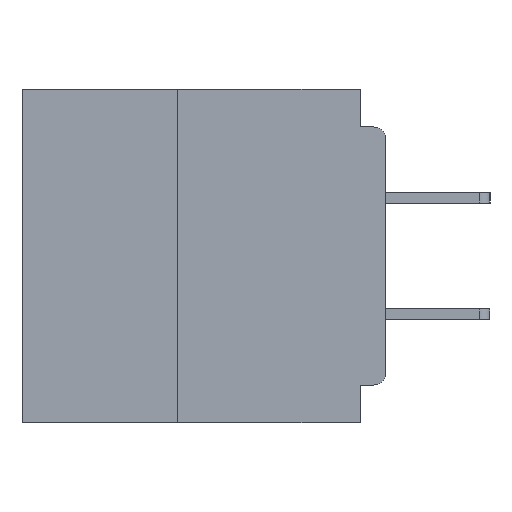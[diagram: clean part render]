
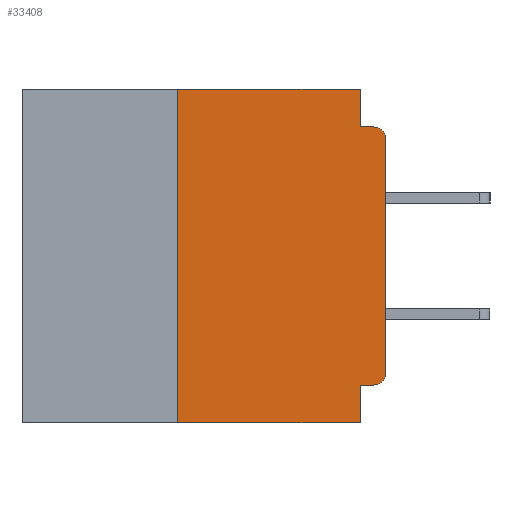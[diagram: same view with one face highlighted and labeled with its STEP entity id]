
A CAD part, left-side view. The second image highlights one B-rep face of the part: STEP entity #33408.
In plain terms, the highlighted planar face has unit normal (-1, 0, 0).
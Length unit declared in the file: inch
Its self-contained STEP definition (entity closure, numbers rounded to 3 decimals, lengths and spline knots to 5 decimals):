
#273 = LINE ( 'NONE', #23625, #36878 ) ;
#636 = VERTEX_POINT ( 'NONE', #52049 ) ;
#1496 = ORIENTED_EDGE ( 'NONE', *, *, #18389, .T. ) ;
#3461 = EDGE_CURVE ( 'NONE', #13959, #16947, #3610, .T. ) ;
#3610 = LINE ( 'NONE', #33844, #27589 ) ;
#4543 = DIRECTION ( 'NONE',  ( 0., -1., 0. ) ) ;
#6542 = DIRECTION ( 'NONE',  ( 0., 1., 0. ) ) ;
#7669 = EDGE_LOOP ( 'NONE', ( #35700, #1496, #8872, #48694, #51312, #60084, #14022, #16538, #50191, #28673 ) ) ;
#8872 = ORIENTED_EDGE ( 'NONE', *, *, #59668, .F. ) ;
#9735 = EDGE_CURVE ( 'NONE', #20068, #16947, #42465, .T. ) ;
#10110 = FACE_OUTER_BOUND ( 'NONE', #7669, .T. ) ;
#12800 = DIRECTION ( 'NONE',  ( 1., 0., 0. ) ) ;
#13531 = LINE ( 'NONE', #49824, #37319 ) ;
#13959 = VERTEX_POINT ( 'NONE', #33513 ) ;
#14022 = ORIENTED_EDGE ( 'NONE', *, *, #9735, .T. ) ;
#16497 = LINE ( 'NONE', #26883, #52813 ) ;
#16538 = ORIENTED_EDGE ( 'NONE', *, *, #3461, .F. ) ;
#16947 = VERTEX_POINT ( 'NONE', #23737 ) ;
#17062 = VERTEX_POINT ( 'NONE', #43379 ) ;
#18389 = EDGE_CURVE ( 'NONE', #31840, #636, #20274, .T. ) ;
#19134 = CARTESIAN_POINT ( 'NONE',  ( 0., 0., -0.06 ) ) ;
#20068 = VERTEX_POINT ( 'NONE', #54970 ) ;
#20274 = CIRCLE ( 'NONE', #51336, 0.015 ) ;
#20973 = AXIS2_PLACEMENT_3D ( 'NONE', #54370, #26064, #59099 ) ;
#22664 = VECTOR ( 'NONE', #28175, 39.37008 ) ;
#22717 = CARTESIAN_POINT ( 'NONE',  ( 0., 0.031, 0. ) ) ;
#23625 = CARTESIAN_POINT ( 'NONE',  ( 0., 0.031, 0. ) ) ;
#23737 = CARTESIAN_POINT ( 'NONE',  ( 0., 0.031, -0.4 ) ) ;
#24056 = CARTESIAN_POINT ( 'NONE',  ( 0., 0., -0.045 ) ) ;
#26064 = DIRECTION ( 'NONE',  ( -1., 0., 0. ) ) ;
#26883 = CARTESIAN_POINT ( 'NONE',  ( 0., 0.437, 0. ) ) ;
#27589 = VECTOR ( 'NONE', #29295, 39.37008 ) ;
#27652 = DIRECTION ( 'NONE',  ( -1., 0., 0. ) ) ;
#28020 = LINE ( 'NONE', #30411, #39096 ) ;
#28175 = DIRECTION ( 'NONE',  ( 0., 0., 1. ) ) ;
#28410 = DIRECTION ( 'NONE',  ( 0., 0., -1. ) ) ;
#28512 = EDGE_CURVE ( 'NONE', #60029, #51605, #16497, .T. ) ;
#28673 = ORIENTED_EDGE ( 'NONE', *, *, #56368, .T. ) ;
#28834 = DIRECTION ( 'NONE',  ( 0., -1., 0. ) ) ;
#29295 = DIRECTION ( 'NONE',  ( 0., 0., -1. ) ) ;
#30411 = CARTESIAN_POINT ( 'NONE',  ( 0., 0., -0.355 ) ) ;
#31840 = VERTEX_POINT ( 'NONE', #19134 ) ;
#33408 = ADVANCED_FACE ( 'NONE', ( #10110 ), #41267, .F. ) ;
#33513 = CARTESIAN_POINT ( 'NONE',  ( 0., 0.031, -0.355 ) ) ;
#33844 = CARTESIAN_POINT ( 'NONE',  ( 0., 0.031, -0.4 ) ) ;
#35251 = LINE ( 'NONE', #46960, #22664 ) ;
#35700 = ORIENTED_EDGE ( 'NONE', *, *, #56002, .T. ) ;
#35819 = DIRECTION ( 'NONE',  ( 0., 0., 1. ) ) ;
#36342 = LINE ( 'NONE', #24056, #47412 ) ;
#36878 = VECTOR ( 'NONE', #28410, 39.37008 ) ;
#37319 = VECTOR ( 'NONE', #35819, 39.37008 ) ;
#38170 = AXIS2_PLACEMENT_3D ( 'NONE', #60080, #12800, #46002 ) ;
#39096 = VECTOR ( 'NONE', #6542, 39.37008 ) ;
#40324 = CARTESIAN_POINT ( 'NONE',  ( 0., 0.015, -0.355 ) ) ;
#40969 = VECTOR ( 'NONE', #4543, 39.37008 ) ;
#41142 = DIRECTION ( 'NONE',  ( 0., -1., 0. ) ) ;
#41267 = PLANE ( 'NONE',  #38170 ) ;
#42433 = VERTEX_POINT ( 'NONE', #50107 ) ;
#42465 = LINE ( 'NONE', #56728, #40969 ) ;
#43379 = CARTESIAN_POINT ( 'NONE',  ( 0., 0.031, -0.045 ) ) ;
#45578 = EDGE_CURVE ( 'NONE', #51605, #17062, #273, .T. ) ;
#46002 = DIRECTION ( 'NONE',  ( 0., 0., -1. ) ) ;
#46960 = CARTESIAN_POINT ( 'NONE',  ( 0., 0., 0. ) ) ;
#47412 = VECTOR ( 'NONE', #28834, 39.37008 ) ;
#47420 = VERTEX_POINT ( 'NONE', #40324 ) ;
#48694 = ORIENTED_EDGE ( 'NONE', *, *, #45578, .F. ) ;
#49824 = CARTESIAN_POINT ( 'NONE',  ( 0., 0.25, -0.4 ) ) ;
#50107 = CARTESIAN_POINT ( 'NONE',  ( 0., 0., -0.34 ) ) ;
#50191 = ORIENTED_EDGE ( 'NONE', *, *, #54805, .F. ) ;
#50708 = CIRCLE ( 'NONE', #20973, 0.015 ) ;
#50923 = EDGE_CURVE ( 'NONE', #20068, #60029, #13531, .T. ) ;
#51312 = ORIENTED_EDGE ( 'NONE', *, *, #28512, .F. ) ;
#51336 = AXIS2_PLACEMENT_3D ( 'NONE', #55979, #27652, #60721 ) ;
#51605 = VERTEX_POINT ( 'NONE', #22717 ) ;
#52049 = CARTESIAN_POINT ( 'NONE',  ( 0., 0.015, -0.045 ) ) ;
#52813 = VECTOR ( 'NONE', #41142, 39.37008 ) ;
#54370 = CARTESIAN_POINT ( 'NONE',  ( 0., 0.015, -0.34 ) ) ;
#54805 = EDGE_CURVE ( 'NONE', #47420, #13959, #28020, .T. ) ;
#54970 = CARTESIAN_POINT ( 'NONE',  ( 0., 0.25, -0.4 ) ) ;
#55979 = CARTESIAN_POINT ( 'NONE',  ( 0., 0.015, -0.06 ) ) ;
#56002 = EDGE_CURVE ( 'NONE', #42433, #31840, #35251, .T. ) ;
#56368 = EDGE_CURVE ( 'NONE', #47420, #42433, #50708, .T. ) ;
#56728 = CARTESIAN_POINT ( 'NONE',  ( 0., 0.437, -0.4 ) ) ;
#59099 = DIRECTION ( 'NONE',  ( 0., 0., -1. ) ) ;
#59668 = EDGE_CURVE ( 'NONE', #17062, #636, #36342, .T. ) ;
#60029 = VERTEX_POINT ( 'NONE', #60617 ) ;
#60080 = CARTESIAN_POINT ( 'NONE',  ( 0., 0.437, 0. ) ) ;
#60084 = ORIENTED_EDGE ( 'NONE', *, *, #50923, .F. ) ;
#60617 = CARTESIAN_POINT ( 'NONE',  ( 0., 0.25, 0. ) ) ;
#60721 = DIRECTION ( 'NONE',  ( 0., 0., -1. ) ) ;
